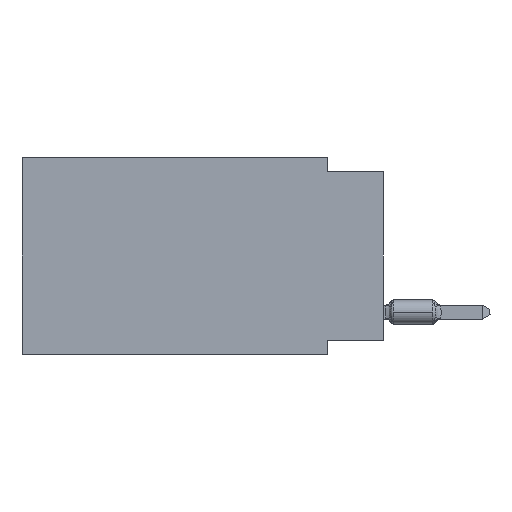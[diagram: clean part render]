
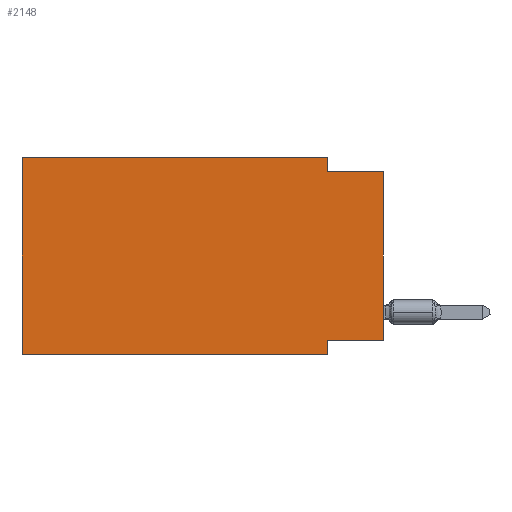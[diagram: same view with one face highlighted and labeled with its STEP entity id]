
A CAD part, left-side view. The second image highlights one B-rep face of the part: STEP entity #2148.
In plain terms, the highlighted planar face has unit normal (-1, 0, 0).
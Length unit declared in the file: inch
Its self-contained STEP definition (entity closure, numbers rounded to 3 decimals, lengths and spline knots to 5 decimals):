
#182 = EDGE_CURVE ( 'NONE', #1995, #5432, #2215, .T. ) ;
#277 = ORIENTED_EDGE ( 'NONE', *, *, #182, .T. ) ;
#773 = VERTEX_POINT ( 'NONE', #15968 ) ;
#1712 = VERTEX_POINT ( 'NONE', #15004 ) ;
#1767 = ORIENTED_EDGE ( 'NONE', *, *, #17838, .T. ) ;
#1792 = CARTESIAN_POINT ( 'NONE',  ( 0., 0.645, 0. ) ) ;
#1908 = VERTEX_POINT ( 'NONE', #11439 ) ;
#1995 = VERTEX_POINT ( 'NONE', #13065 ) ;
#2148 = ADVANCED_FACE ( 'NONE', ( #3912 ), #13521, .F. ) ;
#2215 = LINE ( 'NONE', #16217, #4014 ) ;
#3161 = DIRECTION ( 'NONE',  ( 0., -1., 0. ) ) ;
#3677 = DIRECTION ( 'NONE',  ( 0., -1., 0. ) ) ;
#3912 = FACE_OUTER_BOUND ( 'NONE', #9779, .T. ) ;
#4014 = VECTOR ( 'NONE', #3677, 39.37008 ) ;
#4253 = DIRECTION ( 'NONE',  ( 0., 1., 0. ) ) ;
#4303 = CARTESIAN_POINT ( 'NONE',  ( 0., 0., -0.025 ) ) ;
#4518 = EDGE_CURVE ( 'NONE', #14396, #5920, #15748, .T. ) ;
#4712 = CARTESIAN_POINT ( 'NONE',  ( 0., 0.1, 0. ) ) ;
#5205 = EDGE_CURVE ( 'NONE', #1995, #7584, #17403, .T. ) ;
#5344 = CARTESIAN_POINT ( 'NONE',  ( 0., 0.1, -0.025 ) ) ;
#5432 = VERTEX_POINT ( 'NONE', #15116 ) ;
#5920 = VERTEX_POINT ( 'NONE', #4303 ) ;
#6077 = LINE ( 'NONE', #4712, #17187 ) ;
#6265 = ORIENTED_EDGE ( 'NONE', *, *, #4518, .F. ) ;
#6368 = VECTOR ( 'NONE', #15674, 39.37008 ) ;
#7126 = DIRECTION ( 'NONE',  ( 0., 0., 1. ) ) ;
#7422 = EDGE_CURVE ( 'NONE', #1712, #1908, #8554, .T. ) ;
#7584 = VERTEX_POINT ( 'NONE', #16962 ) ;
#8126 = DIRECTION ( 'NONE',  ( 1., 0., 0. ) ) ;
#8554 = LINE ( 'NONE', #16776, #16808 ) ;
#8846 = ORIENTED_EDGE ( 'NONE', *, *, #11688, .F. ) ;
#9452 = CARTESIAN_POINT ( 'NONE',  ( 0., 0., 0. ) ) ;
#9779 = EDGE_LOOP ( 'NONE', ( #1767, #6265, #8846, #10836, #16165, #277, #10550, #11550 ) ) ;
#10036 = EDGE_CURVE ( 'NONE', #7584, #773, #15531, .T. ) ;
#10084 = VECTOR ( 'NONE', #14365, 39.37008 ) ;
#10101 = LINE ( 'NONE', #10274, #6368 ) ;
#10274 = CARTESIAN_POINT ( 'NONE',  ( 0., 0.1, -0.35 ) ) ;
#10372 = DIRECTION ( 'NONE',  ( 0., 0., -1. ) ) ;
#10550 = ORIENTED_EDGE ( 'NONE', *, *, #17589, .F. ) ;
#10836 = ORIENTED_EDGE ( 'NONE', *, *, #10036, .F. ) ;
#11328 = VECTOR ( 'NONE', #3161, 39.37008 ) ;
#11439 = CARTESIAN_POINT ( 'NONE',  ( 0., 0.1, -0.325 ) ) ;
#11550 = ORIENTED_EDGE ( 'NONE', *, *, #7422, .F. ) ;
#11688 = EDGE_CURVE ( 'NONE', #773, #14396, #6077, .T. ) ;
#12156 = CARTESIAN_POINT ( 'NONE',  ( 0., 0.645, 0. ) ) ;
#13065 = CARTESIAN_POINT ( 'NONE',  ( 0., 0.645, -0.35 ) ) ;
#13193 = DIRECTION ( 'NONE',  ( 0., 0., 1. ) ) ;
#13521 = PLANE ( 'NONE',  #15370 ) ;
#13689 = VECTOR ( 'NONE', #7126, 39.37008 ) ;
#14365 = DIRECTION ( 'NONE',  ( 0., -1., 0. ) ) ;
#14396 = VERTEX_POINT ( 'NONE', #5344 ) ;
#14537 = CARTESIAN_POINT ( 'NONE',  ( 0., 0., -0.025 ) ) ;
#14563 = CARTESIAN_POINT ( 'NONE',  ( 0., 0.645, 0. ) ) ;
#15004 = CARTESIAN_POINT ( 'NONE',  ( 0., 0., -0.325 ) ) ;
#15016 = LINE ( 'NONE', #9452, #13689 ) ;
#15116 = CARTESIAN_POINT ( 'NONE',  ( 0., 0.1, -0.35 ) ) ;
#15370 = AXIS2_PLACEMENT_3D ( 'NONE', #12156, #8126, #17641 ) ;
#15531 = LINE ( 'NONE', #1792, #11328 ) ;
#15674 = DIRECTION ( 'NONE',  ( 0., 0., -1. ) ) ;
#15748 = LINE ( 'NONE', #14537, #10084 ) ;
#15968 = CARTESIAN_POINT ( 'NONE',  ( 0., 0.1, 0. ) ) ;
#16165 = ORIENTED_EDGE ( 'NONE', *, *, #5205, .F. ) ;
#16217 = CARTESIAN_POINT ( 'NONE',  ( 0., 0.645, -0.35 ) ) ;
#16776 = CARTESIAN_POINT ( 'NONE',  ( 0., 0., -0.325 ) ) ;
#16808 = VECTOR ( 'NONE', #4253, 39.37008 ) ;
#16962 = CARTESIAN_POINT ( 'NONE',  ( 0., 0.645, 0. ) ) ;
#17187 = VECTOR ( 'NONE', #10372, 39.37008 ) ;
#17336 = VECTOR ( 'NONE', #13193, 39.37008 ) ;
#17403 = LINE ( 'NONE', #14563, #17336 ) ;
#17589 = EDGE_CURVE ( 'NONE', #1908, #5432, #10101, .T. ) ;
#17641 = DIRECTION ( 'NONE',  ( 0., 0., -1. ) ) ;
#17838 = EDGE_CURVE ( 'NONE', #1712, #5920, #15016, .T. ) ;
